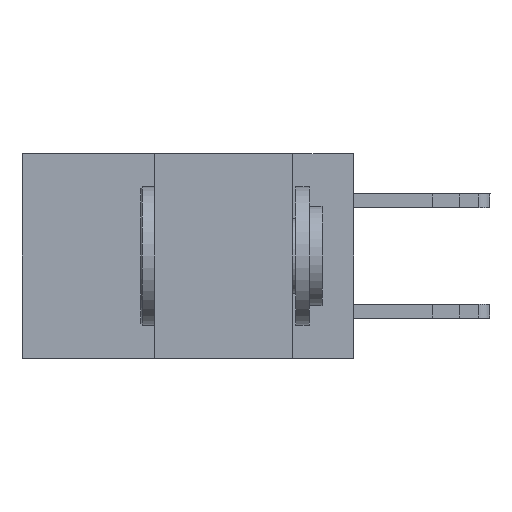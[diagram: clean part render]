
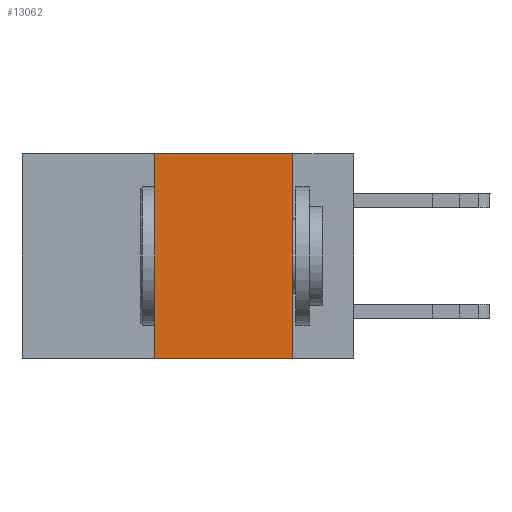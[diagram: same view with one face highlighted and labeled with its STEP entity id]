
A CAD part, left-side view. The second image highlights one B-rep face of the part: STEP entity #13062.
In plain terms, the highlighted planar face has unit normal (-1, 0, 0).
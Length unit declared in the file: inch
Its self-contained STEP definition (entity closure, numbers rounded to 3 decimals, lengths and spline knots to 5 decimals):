
#132 = CARTESIAN_POINT ( 'NONE',  ( 0., 0.11, -0.37 ) ) ;
#308 = VECTOR ( 'NONE', #7963, 39.37008 ) ;
#547 = VERTEX_POINT ( 'NONE', #132 ) ;
#1531 = CARTESIAN_POINT ( 'NONE',  ( 0., 0.36, -0.37 ) ) ;
#2443 = VECTOR ( 'NONE', #15390, 39.37008 ) ;
#2737 = VECTOR ( 'NONE', #8870, 39.37008 ) ;
#2778 = VECTOR ( 'NONE', #5182, 39.37008 ) ;
#3768 = EDGE_CURVE ( 'NONE', #14204, #10542, #6248, .T. ) ;
#4171 = ORIENTED_EDGE ( 'NONE', *, *, #13904, .T. ) ;
#4340 = DIRECTION ( 'NONE',  ( 1., 0., 0. ) ) ;
#5091 = EDGE_CURVE ( 'NONE', #8507, #14204, #16515, .T. ) ;
#5182 = DIRECTION ( 'NONE',  ( 0., -1., 0. ) ) ;
#5240 = ORIENTED_EDGE ( 'NONE', *, *, #5091, .F. ) ;
#5374 = CARTESIAN_POINT ( 'NONE',  ( 0., 0.6, -0.37 ) ) ;
#5391 = AXIS2_PLACEMENT_3D ( 'NONE', #14685, #4340, #13436 ) ;
#6248 = LINE ( 'NONE', #10368, #2778 ) ;
#6287 = EDGE_CURVE ( 'NONE', #10542, #547, #7131, .T. ) ;
#7131 = LINE ( 'NONE', #14090, #2443 ) ;
#7720 = CARTESIAN_POINT ( 'NONE',  ( 0., 0.11, 0. ) ) ;
#7963 = DIRECTION ( 'NONE',  ( 0., -1., 0. ) ) ;
#8507 = VERTEX_POINT ( 'NONE', #1531 ) ;
#8870 = DIRECTION ( 'NONE',  ( 0., 0., 1. ) ) ;
#9875 = LINE ( 'NONE', #5374, #308 ) ;
#10143 = EDGE_LOOP ( 'NONE', ( #16344, #11346, #5240, #4171 ) ) ;
#10368 = CARTESIAN_POINT ( 'NONE',  ( 0., 0.6, 0. ) ) ;
#10542 = VERTEX_POINT ( 'NONE', #7720 ) ;
#10803 = FACE_OUTER_BOUND ( 'NONE', #10143, .T. ) ;
#11346 = ORIENTED_EDGE ( 'NONE', *, *, #3768, .F. ) ;
#12148 = PLANE ( 'NONE',  #5391 ) ;
#13062 = ADVANCED_FACE ( 'NONE', ( #10803 ), #12148, .F. ) ;
#13436 = DIRECTION ( 'NONE',  ( 0., 0., -1. ) ) ;
#13730 = CARTESIAN_POINT ( 'NONE',  ( 0., 0.36, 0. ) ) ;
#13904 = EDGE_CURVE ( 'NONE', #8507, #547, #9875, .T. ) ;
#14068 = CARTESIAN_POINT ( 'NONE',  ( 0., 0.36, 0. ) ) ;
#14090 = CARTESIAN_POINT ( 'NONE',  ( 0., 0.11, 0. ) ) ;
#14204 = VERTEX_POINT ( 'NONE', #13730 ) ;
#14685 = CARTESIAN_POINT ( 'NONE',  ( 0., 0.6, 0. ) ) ;
#15390 = DIRECTION ( 'NONE',  ( 0., 0., -1. ) ) ;
#16344 = ORIENTED_EDGE ( 'NONE', *, *, #6287, .F. ) ;
#16515 = LINE ( 'NONE', #14068, #2737 ) ;
